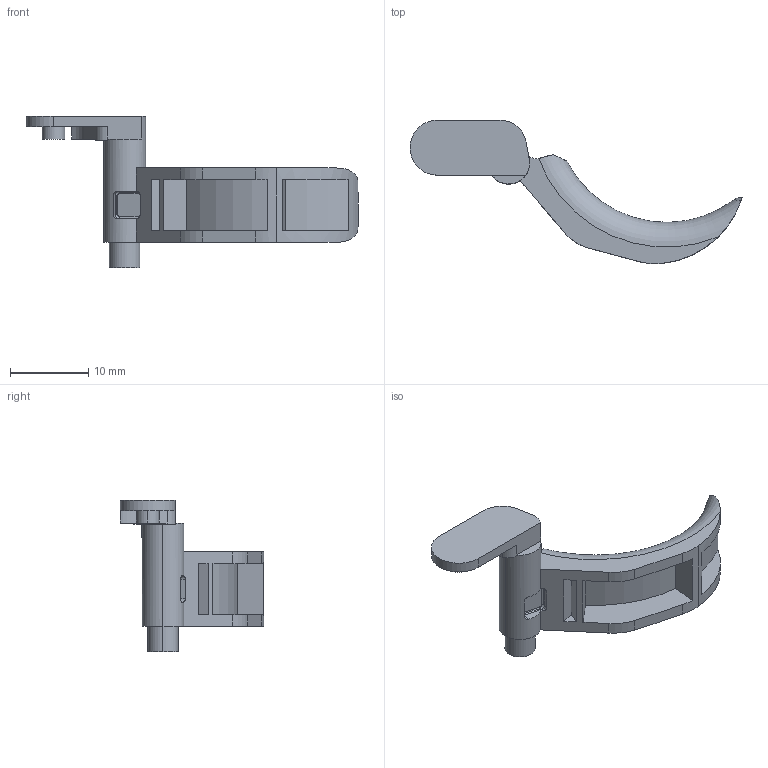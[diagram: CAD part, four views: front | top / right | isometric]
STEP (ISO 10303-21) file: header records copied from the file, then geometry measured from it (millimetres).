
FILE_DESCRIPTION (( 'STEP AP214' ), '1' );
FILE_NAME ('Trigger.step', '2014-07-30T19:47:10', ( 'WarFairy' ), ( '' ), 'SwSTEP 2.0', 'SolidWorks 2013', '' );
FILE_SCHEMA (( 'AUTOMOTIVE_DESIGN' ));
Length unit declared in the file: millimetre
Products named in the file (1): Trigger
Bounding box: 42.46 x 18.34 x 19.37 mm (x, y, z)
Volume: 1435.4 mm3; surface area: 1614.9 mm2
Topology: 1 solids, 1 shells, 78 faces, 208 edges, 135 vertices
Faces by surface type: cylinder 36, plane 34, torus 6, bspline 2
Entity records: 2644 total; most frequent: CARTESIAN_POINT 646, DIRECTION 419, ORIENTED_EDGE 414, EDGE_CURVE 207, AXIS2_PLACEMENT_3D 157, VERTEX_POINT 135, LINE 105, VECTOR 105
